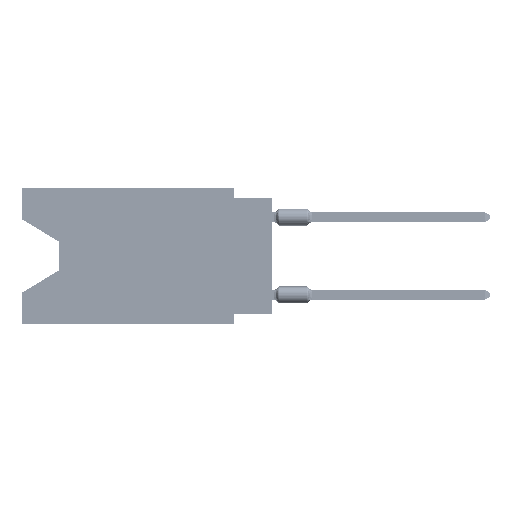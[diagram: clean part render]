
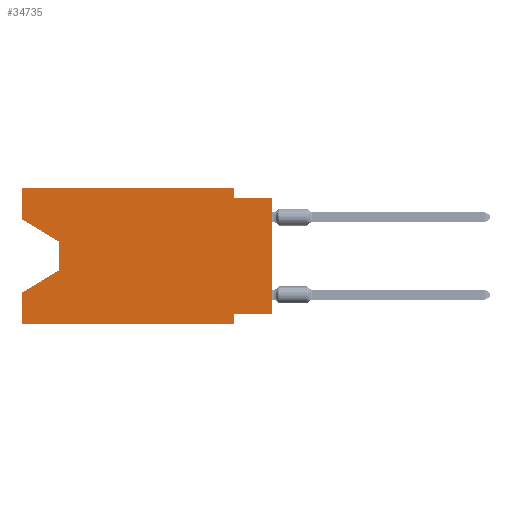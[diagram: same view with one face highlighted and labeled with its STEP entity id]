
A CAD part, left-side view. The second image highlights one B-rep face of the part: STEP entity #34735.
In plain terms, the highlighted planar face has unit normal (-1, 0, 0).
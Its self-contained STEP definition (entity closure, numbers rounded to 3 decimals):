
#656 = EDGE_CURVE ( 'NONE', #50133, #82372, #34630, .T. ) ;
#872 = VECTOR ( 'NONE', #63244, 1000. ) ;
#2201 = VERTEX_POINT ( 'NONE', #49118 ) ;
#2485 = VECTOR ( 'NONE', #53560, 1000. ) ;
#5352 = VERTEX_POINT ( 'NONE', #53370 ) ;
#6154 = EDGE_CURVE ( 'NONE', #82392, #35595, #9323, .T. ) ;
#7152 = VERTEX_POINT ( 'NONE', #44082 ) ;
#8907 = VECTOR ( 'NONE', #22167, 1000. ) ;
#9323 = LINE ( 'NONE', #67572, #8907 ) ;
#9371 = VECTOR ( 'NONE', #49522, 1000. ) ;
#9905 = CARTESIAN_POINT ( 'NONE',  ( 0., 2.54, 0. ) ) ;
#9910 = VECTOR ( 'NONE', #43508, 1000. ) ;
#10518 = EDGE_CURVE ( 'NONE', #2201, #7152, #36702, .T. ) ;
#11534 = CARTESIAN_POINT ( 'NONE',  ( 0., 16.383, -6.852 ) ) ;
#12438 = EDGE_CURVE ( 'NONE', #30355, #20113, #13464, .T. ) ;
#13464 = LINE ( 'NONE', #59278, #24422 ) ;
#13783 = EDGE_CURVE ( 'NONE', #5352, #56168, #50378, .T. ) ;
#13792 = LINE ( 'NONE', #20628, #52124 ) ;
#14189 = LINE ( 'NONE', #41969, #2485 ) ;
#15821 = DIRECTION ( 'NONE',  ( 0., 0., -1. ) ) ;
#16445 = ORIENTED_EDGE ( 'NONE', *, *, #51796, .F. ) ;
#16660 = DIRECTION ( 'NONE',  ( 1., 0., 0. ) ) ;
#17402 = CARTESIAN_POINT ( 'NONE',  ( 0., 2.54, 0. ) ) ;
#17495 = CARTESIAN_POINT ( 'NONE',  ( 0., 2.54, -8.255 ) ) ;
#17797 = ORIENTED_EDGE ( 'NONE', *, *, #12438, .F. ) ;
#18273 = DIRECTION ( 'NONE',  ( 0., -0.855, -0.519 ) ) ;
#18683 = CARTESIAN_POINT ( 'NONE',  ( 0., 16.383, -2.038 ) ) ;
#20113 = VERTEX_POINT ( 'NONE', #11534 ) ;
#20429 = ORIENTED_EDGE ( 'NONE', *, *, #656, .F. ) ;
#20628 = CARTESIAN_POINT ( 'NONE',  ( 0., 13.97, -3.505 ) ) ;
#21397 = LINE ( 'NONE', #45820, #41414 ) ;
#21472 = AXIS2_PLACEMENT_3D ( 'NONE', #68896, #16660, #15821 ) ;
#21515 = VECTOR ( 'NONE', #82451, 1000. ) ;
#22167 = DIRECTION ( 'NONE',  ( 0., -1., 0. ) ) ;
#22196 = EDGE_CURVE ( 'NONE', #46504, #7152, #74366, .T. ) ;
#23010 = CARTESIAN_POINT ( 'NONE',  ( 0., 16.383, 0. ) ) ;
#23977 = CARTESIAN_POINT ( 'NONE',  ( 0., 13.97, -5.385 ) ) ;
#24422 = VECTOR ( 'NONE', #65683, 1000. ) ;
#26127 = DIRECTION ( 'NONE',  ( 0., 1., 0. ) ) ;
#27957 = ORIENTED_EDGE ( 'NONE', *, *, #70051, .F. ) ;
#29286 = ORIENTED_EDGE ( 'NONE', *, *, #10518, .F. ) ;
#29508 = EDGE_LOOP ( 'NONE', ( #46767, #36327, #68626, #17797, #71078, #20429, #27957, #64810, #29286, #16445, #61234, #65579 ) ) ;
#30355 = VERTEX_POINT ( 'NONE', #53428 ) ;
#34630 = LINE ( 'NONE', #79998, #76817 ) ;
#34735 = ADVANCED_FACE ( 'NONE', ( #67206 ), #60788, .F. ) ;
#35595 = VERTEX_POINT ( 'NONE', #9905 ) ;
#36327 = ORIENTED_EDGE ( 'NONE', *, *, #66290, .T. ) ;
#36702 = LINE ( 'NONE', #61560, #872 ) ;
#37642 = CARTESIAN_POINT ( 'NONE',  ( 0., 0., -8.255 ) ) ;
#41414 = VECTOR ( 'NONE', #26127, 1000. ) ;
#41969 = CARTESIAN_POINT ( 'NONE',  ( 0., 16.383, -8.89 ) ) ;
#42732 = DIRECTION ( 'NONE',  ( 0., 0., -1. ) ) ;
#43508 = DIRECTION ( 'NONE',  ( 0., 0., -1. ) ) ;
#44082 = CARTESIAN_POINT ( 'NONE',  ( 0., 0., -0.635 ) ) ;
#45097 = LINE ( 'NONE', #23010, #9371 ) ;
#45605 = EDGE_CURVE ( 'NONE', #5352, #82392, #45097, .T. ) ;
#45820 = CARTESIAN_POINT ( 'NONE',  ( 0., 0., -8.255 ) ) ;
#46480 = CARTESIAN_POINT ( 'NONE',  ( 0., 2.54, -8.89 ) ) ;
#46504 = VERTEX_POINT ( 'NONE', #37642 ) ;
#46767 = ORIENTED_EDGE ( 'NONE', *, *, #13783, .T. ) ;
#48593 = CARTESIAN_POINT ( 'NONE',  ( 0., 16.383, 0. ) ) ;
#49118 = CARTESIAN_POINT ( 'NONE',  ( 0., 2.54, -0.635 ) ) ;
#49522 = DIRECTION ( 'NONE',  ( 0., 0., 1. ) ) ;
#50133 = VERTEX_POINT ( 'NONE', #17495 ) ;
#50378 = LINE ( 'NONE', #18683, #64336 ) ;
#51796 = EDGE_CURVE ( 'NONE', #35595, #2201, #61957, .T. ) ;
#52124 = VECTOR ( 'NONE', #59594, 1000. ) ;
#53370 = CARTESIAN_POINT ( 'NONE',  ( 0., 16.383, -2.038 ) ) ;
#53428 = CARTESIAN_POINT ( 'NONE',  ( 0., 16.383, -8.89 ) ) ;
#53560 = DIRECTION ( 'NONE',  ( 0., -1., 0. ) ) ;
#56168 = VERTEX_POINT ( 'NONE', #68335 ) ;
#56350 = CARTESIAN_POINT ( 'NONE',  ( 0., 0., 0. ) ) ;
#59278 = CARTESIAN_POINT ( 'NONE',  ( 0., 16.383, 0. ) ) ;
#59594 = DIRECTION ( 'NONE',  ( 0., 0., -1. ) ) ;
#60788 = PLANE ( 'NONE',  #21472 ) ;
#61234 = ORIENTED_EDGE ( 'NONE', *, *, #6154, .F. ) ;
#61560 = CARTESIAN_POINT ( 'NONE',  ( 0., 0., -0.635 ) ) ;
#61957 = LINE ( 'NONE', #17402, #9910 ) ;
#62840 = CARTESIAN_POINT ( 'NONE',  ( 0., 13.97, -5.385 ) ) ;
#63244 = DIRECTION ( 'NONE',  ( 0., -1., 0. ) ) ;
#63276 = EDGE_CURVE ( 'NONE', #75505, #20113, #76527, .T. ) ;
#63687 = DIRECTION ( 'NONE',  ( 0., 0.855, -0.519 ) ) ;
#64067 = VECTOR ( 'NONE', #63687, 1000. ) ;
#64336 = VECTOR ( 'NONE', #18273, 1000. ) ;
#64810 = ORIENTED_EDGE ( 'NONE', *, *, #22196, .T. ) ;
#65579 = ORIENTED_EDGE ( 'NONE', *, *, #45605, .F. ) ;
#65683 = DIRECTION ( 'NONE',  ( 0., 0., 1. ) ) ;
#66290 = EDGE_CURVE ( 'NONE', #56168, #75505, #13792, .T. ) ;
#67206 = FACE_OUTER_BOUND ( 'NONE', #29508, .T. ) ;
#67572 = CARTESIAN_POINT ( 'NONE',  ( 0., 16.383, 0. ) ) ;
#68335 = CARTESIAN_POINT ( 'NONE',  ( 0., 13.97, -3.505 ) ) ;
#68626 = ORIENTED_EDGE ( 'NONE', *, *, #63276, .T. ) ;
#68896 = CARTESIAN_POINT ( 'NONE',  ( 0., 16.383, 0. ) ) ;
#70051 = EDGE_CURVE ( 'NONE', #46504, #50133, #21397, .T. ) ;
#71078 = ORIENTED_EDGE ( 'NONE', *, *, #72982, .T. ) ;
#72982 = EDGE_CURVE ( 'NONE', #30355, #82372, #14189, .T. ) ;
#74366 = LINE ( 'NONE', #56350, #21515 ) ;
#75505 = VERTEX_POINT ( 'NONE', #23977 ) ;
#76527 = LINE ( 'NONE', #62840, #64067 ) ;
#76817 = VECTOR ( 'NONE', #42732, 1000. ) ;
#79998 = CARTESIAN_POINT ( 'NONE',  ( 0., 2.54, -8.89 ) ) ;
#82372 = VERTEX_POINT ( 'NONE', #46480 ) ;
#82392 = VERTEX_POINT ( 'NONE', #48593 ) ;
#82451 = DIRECTION ( 'NONE',  ( 0., 0., 1. ) ) ;
